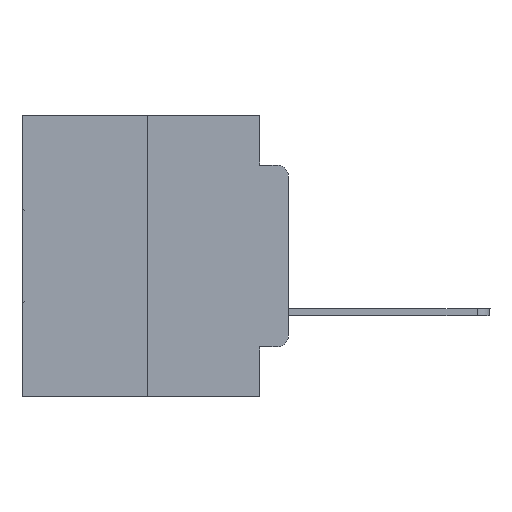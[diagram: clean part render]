
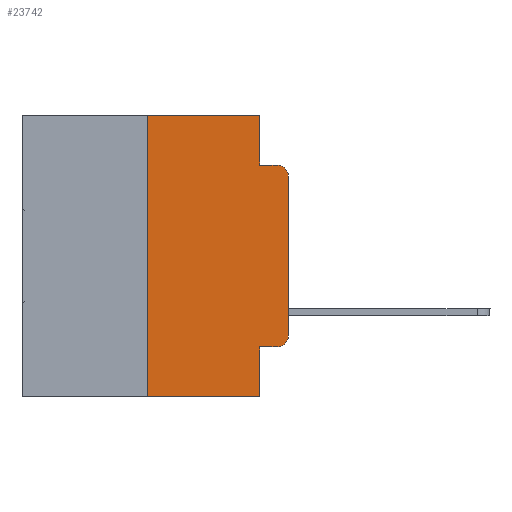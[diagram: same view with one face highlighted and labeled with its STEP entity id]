
A CAD part, left-side view. The second image highlights one B-rep face of the part: STEP entity #23742.
In plain terms, the highlighted planar face has unit normal (-1, 0, 0).
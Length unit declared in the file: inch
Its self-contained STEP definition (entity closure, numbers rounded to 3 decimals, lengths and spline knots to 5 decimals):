
#524 = CARTESIAN_POINT ( 'NONE',  ( 0., 0.051, 0. ) ) ;
#605 = ORIENTED_EDGE ( 'NONE', *, *, #11936, .F. ) ;
#615 = ORIENTED_EDGE ( 'NONE', *, *, #3450, .F. ) ;
#868 = VECTOR ( 'NONE', #13134, 39.37008 ) ;
#1044 = LINE ( 'NONE', #27017, #23569 ) ;
#1805 = EDGE_LOOP ( 'NONE', ( #11276, #27031, #21474, #605, #6969, #30288, #19415, #615, #4989, #17934 ) ) ;
#1825 = FACE_OUTER_BOUND ( 'NONE', #1805, .T. ) ;
#1977 = DIRECTION ( 'NONE',  ( 0., 0., -1. ) ) ;
#2780 = AXIS2_PLACEMENT_3D ( 'NONE', #15865, #4257, #25875 ) ;
#3450 = EDGE_CURVE ( 'NONE', #28903, #13791, #6309, .T. ) ;
#3960 = VERTEX_POINT ( 'NONE', #20604 ) ;
#4010 = CARTESIAN_POINT ( 'NONE',  ( 0., 0.02, -0.4115 ) ) ;
#4142 = LINE ( 'NONE', #6311, #6865 ) ;
#4257 = DIRECTION ( 'NONE',  ( -1., 0., 0. ) ) ;
#4668 = CARTESIAN_POINT ( 'NONE',  ( 0., 0.25, 0. ) ) ;
#4989 = ORIENTED_EDGE ( 'NONE', *, *, #7914, .T. ) ;
#5469 = VECTOR ( 'NONE', #29112, 39.37008 ) ;
#5649 = CARTESIAN_POINT ( 'NONE',  ( 0., 0., -0.3915 ) ) ;
#5930 = CARTESIAN_POINT ( 'NONE',  ( 0., 0.25, 0. ) ) ;
#6198 = VERTEX_POINT ( 'NONE', #4010 ) ;
#6309 = LINE ( 'NONE', #18063, #868 ) ;
#6311 = CARTESIAN_POINT ( 'NONE',  ( 0., 0.473, 0. ) ) ;
#6865 = VECTOR ( 'NONE', #20685, 39.37008 ) ;
#6969 = ORIENTED_EDGE ( 'NONE', *, *, #30472, .F. ) ;
#7088 = AXIS2_PLACEMENT_3D ( 'NONE', #8951, #20693, #1977 ) ;
#7914 = EDGE_CURVE ( 'NONE', #28903, #6198, #1044, .T. ) ;
#8053 = CIRCLE ( 'NONE', #25365, 0.02 ) ;
#8288 = VERTEX_POINT ( 'NONE', #5649 ) ;
#8340 = VERTEX_POINT ( 'NONE', #20028 ) ;
#8728 = LINE ( 'NONE', #18002, #19570 ) ;
#8740 = EDGE_CURVE ( 'NONE', #6198, #8288, #8053, .T. ) ;
#8951 = CARTESIAN_POINT ( 'NONE',  ( 0., 0.473, 0. ) ) ;
#9286 = EDGE_CURVE ( 'NONE', #3960, #20271, #14420, .T. ) ;
#10345 = CARTESIAN_POINT ( 'NONE',  ( 0., 0.051, -0.0885 ) ) ;
#10347 = CARTESIAN_POINT ( 'NONE',  ( 0., 0.051, -0.4115 ) ) ;
#10501 = CARTESIAN_POINT ( 'NONE',  ( 0., 0.02, -0.0885 ) ) ;
#10576 = CARTESIAN_POINT ( 'NONE',  ( 0., 0.051, -0.5 ) ) ;
#10687 = CIRCLE ( 'NONE', #2780, 0.02 ) ;
#11276 = ORIENTED_EDGE ( 'NONE', *, *, #14081, .T. ) ;
#11535 = CARTESIAN_POINT ( 'NONE',  ( 0., 0., -0.1085 ) ) ;
#11788 = DIRECTION ( 'NONE',  ( 0., 0., 1. ) ) ;
#11936 = EDGE_CURVE ( 'NONE', #16738, #8340, #17231, .T. ) ;
#12371 = DIRECTION ( 'NONE',  ( 0., -1., 0. ) ) ;
#13134 = DIRECTION ( 'NONE',  ( 0., 0., -1. ) ) ;
#13288 = DIRECTION ( 'NONE',  ( 0., -1., 0. ) ) ;
#13791 = VERTEX_POINT ( 'NONE', #10576 ) ;
#14081 = EDGE_CURVE ( 'NONE', #8288, #19999, #23784, .T. ) ;
#14420 = LINE ( 'NONE', #4668, #15836 ) ;
#14554 = DIRECTION ( 'NONE',  ( 0., 0., 1. ) ) ;
#14706 = CARTESIAN_POINT ( 'NONE',  ( 0., 0., 0. ) ) ;
#15836 = VECTOR ( 'NONE', #11788, 39.37008 ) ;
#15865 = CARTESIAN_POINT ( 'NONE',  ( 0., 0.02, -0.1085 ) ) ;
#15955 = VECTOR ( 'NONE', #14554, 39.37008 ) ;
#16738 = VERTEX_POINT ( 'NONE', #17893 ) ;
#17231 = LINE ( 'NONE', #524, #5469 ) ;
#17893 = CARTESIAN_POINT ( 'NONE',  ( 0., 0.051, 0. ) ) ;
#17934 = ORIENTED_EDGE ( 'NONE', *, *, #8740, .T. ) ;
#17995 = EDGE_CURVE ( 'NONE', #8340, #19236, #19622, .T. ) ;
#18002 = CARTESIAN_POINT ( 'NONE',  ( 0., 0.473, -0.5 ) ) ;
#18054 = VECTOR ( 'NONE', #12371, 39.37008 ) ;
#18063 = CARTESIAN_POINT ( 'NONE',  ( 0., 0.051, 0. ) ) ;
#18716 = EDGE_CURVE ( 'NONE', #19999, #19236, #10687, .T. ) ;
#18774 = CARTESIAN_POINT ( 'NONE',  ( 0., 0.02, -0.3915 ) ) ;
#19236 = VERTEX_POINT ( 'NONE', #10501 ) ;
#19415 = ORIENTED_EDGE ( 'NONE', *, *, #28033, .T. ) ;
#19570 = VECTOR ( 'NONE', #25237, 39.37008 ) ;
#19622 = LINE ( 'NONE', #10345, #18054 ) ;
#19999 = VERTEX_POINT ( 'NONE', #11535 ) ;
#20028 = CARTESIAN_POINT ( 'NONE',  ( 0., 0.051, -0.0885 ) ) ;
#20271 = VERTEX_POINT ( 'NONE', #5930 ) ;
#20604 = CARTESIAN_POINT ( 'NONE',  ( 0., 0.25, -0.5 ) ) ;
#20685 = DIRECTION ( 'NONE',  ( 0., -1., 0. ) ) ;
#20693 = DIRECTION ( 'NONE',  ( 1., 0., 0. ) ) ;
#21474 = ORIENTED_EDGE ( 'NONE', *, *, #17995, .F. ) ;
#23569 = VECTOR ( 'NONE', #13288, 39.37008 ) ;
#23742 = ADVANCED_FACE ( 'NONE', ( #1825 ), #29231, .F. ) ;
#23784 = LINE ( 'NONE', #14706, #15955 ) ;
#25237 = DIRECTION ( 'NONE',  ( 0., -1., 0. ) ) ;
#25365 = AXIS2_PLACEMENT_3D ( 'NONE', #18774, #28184, #25393 ) ;
#25393 = DIRECTION ( 'NONE',  ( 0., 0., -1. ) ) ;
#25875 = DIRECTION ( 'NONE',  ( 0., 0., -1. ) ) ;
#27017 = CARTESIAN_POINT ( 'NONE',  ( 0., 0.051, -0.4115 ) ) ;
#27031 = ORIENTED_EDGE ( 'NONE', *, *, #18716, .T. ) ;
#28033 = EDGE_CURVE ( 'NONE', #3960, #13791, #8728, .T. ) ;
#28184 = DIRECTION ( 'NONE',  ( -1., 0., 0. ) ) ;
#28903 = VERTEX_POINT ( 'NONE', #10347 ) ;
#29112 = DIRECTION ( 'NONE',  ( 0., 0., -1. ) ) ;
#29231 = PLANE ( 'NONE',  #7088 ) ;
#30288 = ORIENTED_EDGE ( 'NONE', *, *, #9286, .F. ) ;
#30472 = EDGE_CURVE ( 'NONE', #20271, #16738, #4142, .T. ) ;
